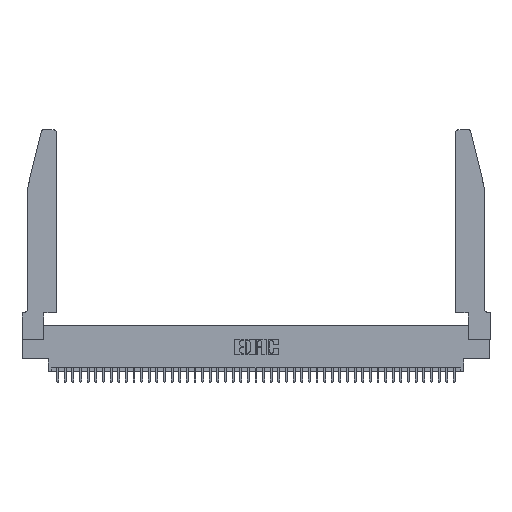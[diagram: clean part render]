
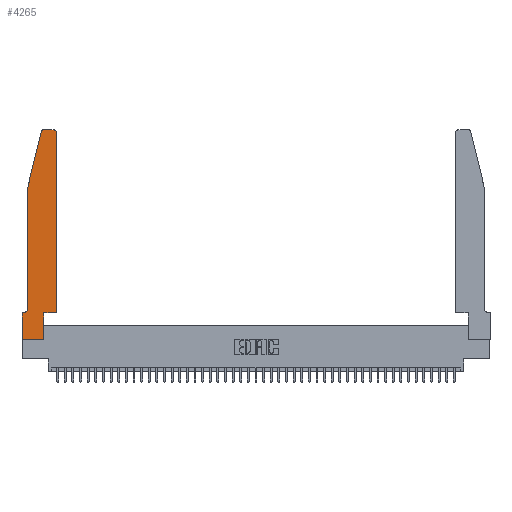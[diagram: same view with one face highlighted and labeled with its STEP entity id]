
A CAD part, top view. The second image highlights one B-rep face of the part: STEP entity #4265.
In plain terms, the highlighted planar face has unit normal (0, 0, 1).
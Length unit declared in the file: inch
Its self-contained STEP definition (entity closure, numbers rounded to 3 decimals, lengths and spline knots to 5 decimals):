
#492 = ORIENTED_EDGE ( 'NONE', *, *, #32319, .T. ) ;
#1149 = DIRECTION ( 'NONE',  ( -1., 0., 0. ) ) ;
#1366 = CARTESIAN_POINT ( 'NONE',  ( 0.4505, 2.72, 0.37 ) ) ;
#1547 = EDGE_CURVE ( 'NONE', #35984, #33624, #14247, .T. ) ;
#2242 = VECTOR ( 'NONE', #40176, 39.37008 ) ;
#2247 = CARTESIAN_POINT ( 'NONE',  ( 0.0755, 2., 0.37 ) ) ;
#2727 = ORIENTED_EDGE ( 'NONE', *, *, #18818, .T. ) ;
#4265 = ADVANCED_FACE ( 'NONE', ( #24873 ), #36439, .T. ) ;
#4731 = LINE ( 'NONE', #17543, #28712 ) ;
#5420 = CIRCLE ( 'NONE', #20407, 0.03 ) ;
#5698 = LINE ( 'NONE', #28718, #26366 ) ;
#6431 = CIRCLE ( 'NONE', #15382, 0.07 ) ;
#7009 = EDGE_CURVE ( 'NONE', #37253, #34122, #18029, .T. ) ;
#7566 = EDGE_CURVE ( 'NONE', #26020, #37253, #5420, .T. ) ;
#7705 = EDGE_LOOP ( 'NONE', ( #40515, #35776, #40521, #35732, #38499, #492, #38376, #2727, #23980, #23333, #37296, #11648 ) ) ;
#7824 = VERTEX_POINT ( 'NONE', #16627 ) ;
#7888 = CARTESIAN_POINT ( 'NONE',  ( 0., 0., 0.37 ) ) ;
#7981 = LINE ( 'NONE', #15056, #9640 ) ;
#8310 = CARTESIAN_POINT ( 'NONE',  ( 0.4505, 0.35, 0.37 ) ) ;
#8334 = CARTESIAN_POINT ( 'NONE',  ( 0.2865, 0.35, 0.37 ) ) ;
#8454 = DIRECTION ( 'NONE',  ( -0.239, -0.971, 0. ) ) ;
#8467 = CARTESIAN_POINT ( 'NONE',  ( 0.0055, 0.42, 0.37 ) ) ;
#8520 = DIRECTION ( 'NONE',  ( 1., 0., 0. ) ) ;
#8764 = CARTESIAN_POINT ( 'NONE',  ( 0.0755, 2., 0.37 ) ) ;
#9423 = CARTESIAN_POINT ( 'NONE',  ( 0.4205, 2.72, 0.37 ) ) ;
#9602 = EDGE_CURVE ( 'NONE', #19028, #22249, #7981, .T. ) ;
#9640 = VECTOR ( 'NONE', #15682, 39.37008 ) ;
#11285 = CARTESIAN_POINT ( 'NONE',  ( 0., 0., 0.37 ) ) ;
#11535 = VERTEX_POINT ( 'NONE', #35271 ) ;
#11642 = DIRECTION ( 'NONE',  ( 0., 0., 1. ) ) ;
#11648 = ORIENTED_EDGE ( 'NONE', *, *, #42729, .T. ) ;
#11996 = CARTESIAN_POINT ( 'NONE',  ( 0.284, 2.72, 0.37 ) ) ;
#14199 = DIRECTION ( 'NONE',  ( 1., 0., 0. ) ) ;
#14247 = LINE ( 'NONE', #8310, #20260 ) ;
#15056 = CARTESIAN_POINT ( 'NONE',  ( 0., 0., 0.37 ) ) ;
#15150 = CARTESIAN_POINT ( 'NONE',  ( 0.2605, 2.75, 0.37 ) ) ;
#15382 = AXIS2_PLACEMENT_3D ( 'NONE', #8467, #28726, #1149 ) ;
#15682 = DIRECTION ( 'NONE',  ( 0., -1., 0. ) ) ;
#16627 = CARTESIAN_POINT ( 'NONE',  ( 0.0755, 0.42, 0.37 ) ) ;
#16924 = VECTOR ( 'NONE', #22171, 39.37008 ) ;
#17543 = CARTESIAN_POINT ( 'NONE',  ( 0.4505, 0.35, 0.37 ) ) ;
#18029 = LINE ( 'NONE', #8764, #44822 ) ;
#18818 = EDGE_CURVE ( 'NONE', #22249, #40059, #30806, .T. ) ;
#19028 = VERTEX_POINT ( 'NONE', #44193 ) ;
#19319 = DIRECTION ( 'NONE',  ( 0., 0., 1. ) ) ;
#19359 = LINE ( 'NONE', #43090, #29206 ) ;
#19840 = VERTEX_POINT ( 'NONE', #20027 ) ;
#20027 = CARTESIAN_POINT ( 'NONE',  ( 0.2865, 0.35, 0.37 ) ) ;
#20260 = VECTOR ( 'NONE', #31292, 39.37008 ) ;
#20407 = AXIS2_PLACEMENT_3D ( 'NONE', #11996, #43289, #39916 ) ;
#20709 = LINE ( 'NONE', #8334, #2242 ) ;
#22050 = VECTOR ( 'NONE', #8520, 39.37008 ) ;
#22171 = DIRECTION ( 'NONE',  ( -1., 0., 0. ) ) ;
#22180 = DIRECTION ( 'NONE',  ( 1., 0., 0. ) ) ;
#22249 = VERTEX_POINT ( 'NONE', #11285 ) ;
#23333 = ORIENTED_EDGE ( 'NONE', *, *, #41806, .T. ) ;
#23980 = ORIENTED_EDGE ( 'NONE', *, *, #39575, .T. ) ;
#24873 = FACE_OUTER_BOUND ( 'NONE', #7705, .T. ) ;
#25962 = CARTESIAN_POINT ( 'NONE',  ( 0.284, 2.75, 0.37 ) ) ;
#26020 = VERTEX_POINT ( 'NONE', #25962 ) ;
#26142 = AXIS2_PLACEMENT_3D ( 'NONE', #38373, #11642, #22180 ) ;
#26366 = VECTOR ( 'NONE', #32219, 39.37008 ) ;
#28712 = VECTOR ( 'NONE', #14199, 39.37008 ) ;
#28718 = CARTESIAN_POINT ( 'NONE',  ( 0.0755, 0.35, 0.37 ) ) ;
#28726 = DIRECTION ( 'NONE',  ( 0., 0., -1. ) ) ;
#29206 = VECTOR ( 'NONE', #36204, 39.37008 ) ;
#29769 = EDGE_CURVE ( 'NONE', #7824, #40475, #6431, .T. ) ;
#30578 = LINE ( 'NONE', #15150, #16924 ) ;
#30806 = LINE ( 'NONE', #7888, #22050 ) ;
#31292 = DIRECTION ( 'NONE',  ( 0., 1., 0. ) ) ;
#32219 = DIRECTION ( 'NONE',  ( -1., 0., 0. ) ) ;
#32319 = EDGE_CURVE ( 'NONE', #40475, #19028, #5698, .T. ) ;
#32959 = CIRCLE ( 'NONE', #44982, 0.03 ) ;
#33624 = VERTEX_POINT ( 'NONE', #1366 ) ;
#34122 = VERTEX_POINT ( 'NONE', #2247 ) ;
#35271 = CARTESIAN_POINT ( 'NONE',  ( 0.4205, 2.75, 0.37 ) ) ;
#35732 = ORIENTED_EDGE ( 'NONE', *, *, #42530, .T. ) ;
#35776 = ORIENTED_EDGE ( 'NONE', *, *, #7566, .T. ) ;
#35932 = CARTESIAN_POINT ( 'NONE',  ( 0.2865, 0., 0.37 ) ) ;
#35984 = VERTEX_POINT ( 'NONE', #38144 ) ;
#36204 = DIRECTION ( 'NONE',  ( 0., -1., 0. ) ) ;
#36439 = PLANE ( 'NONE',  #26142 ) ;
#37145 = DIRECTION ( 'NONE',  ( 1., 0., 0. ) ) ;
#37253 = VERTEX_POINT ( 'NONE', #44653 ) ;
#37296 = ORIENTED_EDGE ( 'NONE', *, *, #1547, .T. ) ;
#38144 = CARTESIAN_POINT ( 'NONE',  ( 0.4505, 0.35, 0.37 ) ) ;
#38373 = CARTESIAN_POINT ( 'NONE',  ( 0., 0.35, 0.37 ) ) ;
#38376 = ORIENTED_EDGE ( 'NONE', *, *, #9602, .T. ) ;
#38499 = ORIENTED_EDGE ( 'NONE', *, *, #29769, .T. ) ;
#39442 = EDGE_CURVE ( 'NONE', #11535, #26020, #30578, .T. ) ;
#39575 = EDGE_CURVE ( 'NONE', #40059, #19840, #20709, .T. ) ;
#39916 = DIRECTION ( 'NONE',  ( 1., 0., 0. ) ) ;
#40059 = VERTEX_POINT ( 'NONE', #35932 ) ;
#40176 = DIRECTION ( 'NONE',  ( 0., 1., 0. ) ) ;
#40475 = VERTEX_POINT ( 'NONE', #41871 ) ;
#40515 = ORIENTED_EDGE ( 'NONE', *, *, #39442, .T. ) ;
#40521 = ORIENTED_EDGE ( 'NONE', *, *, #7009, .T. ) ;
#41806 = EDGE_CURVE ( 'NONE', #19840, #35984, #4731, .T. ) ;
#41871 = CARTESIAN_POINT ( 'NONE',  ( 0.0055, 0.35, 0.37 ) ) ;
#42530 = EDGE_CURVE ( 'NONE', #34122, #7824, #19359, .T. ) ;
#42729 = EDGE_CURVE ( 'NONE', #33624, #11535, #32959, .T. ) ;
#43090 = CARTESIAN_POINT ( 'NONE',  ( 0.0755, 2., 0.37 ) ) ;
#43289 = DIRECTION ( 'NONE',  ( 0., 0., 1. ) ) ;
#44193 = CARTESIAN_POINT ( 'NONE',  ( 0., 0.35, 0.37 ) ) ;
#44653 = CARTESIAN_POINT ( 'NONE',  ( 0.25487, 2.72718, 0.37 ) ) ;
#44822 = VECTOR ( 'NONE', #8454, 39.37008 ) ;
#44982 = AXIS2_PLACEMENT_3D ( 'NONE', #9423, #19319, #37145 ) ;
